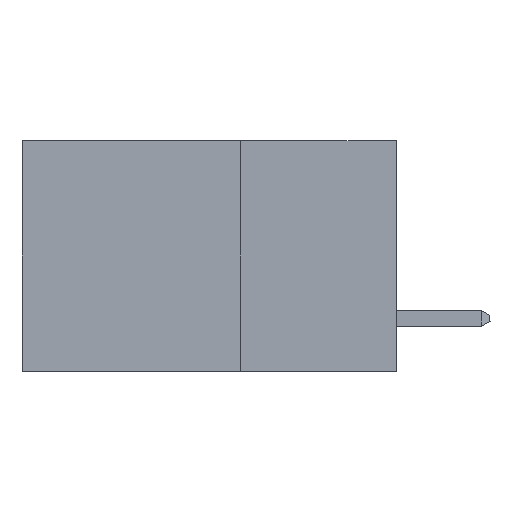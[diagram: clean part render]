
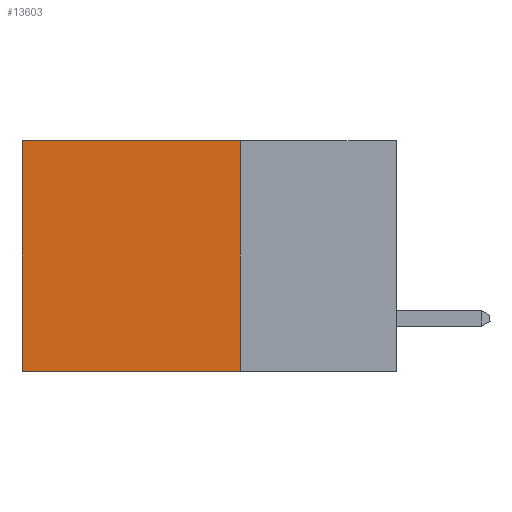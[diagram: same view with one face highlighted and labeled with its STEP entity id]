
A CAD part, left-side view. The second image highlights one B-rep face of the part: STEP entity #13603.
In plain terms, the highlighted planar face has unit normal (-1, 0, 0).
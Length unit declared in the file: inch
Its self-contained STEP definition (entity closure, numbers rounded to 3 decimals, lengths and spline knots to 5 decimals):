
#178 = VECTOR ( 'NONE', #5816, 39.37008 ) ;
#515 = EDGE_CURVE ( 'NONE', #1883, #13728, #14720, .T. ) ;
#1825 = VECTOR ( 'NONE', #14059, 39.37008 ) ;
#1883 = VERTEX_POINT ( 'NONE', #7323 ) ;
#2165 = CARTESIAN_POINT ( 'NONE',  ( 0.298, 0.6, -0.37 ) ) ;
#3033 = LINE ( 'NONE', #6489, #6186 ) ;
#3456 = EDGE_LOOP ( 'NONE', ( #7379, #7427, #7745, #8244 ) ) ;
#3916 = CARTESIAN_POINT ( 'NONE',  ( 0.298, 0.6, 0. ) ) ;
#4239 = CARTESIAN_POINT ( 'NONE',  ( 0.298, 0.6, 0. ) ) ;
#4866 = VECTOR ( 'NONE', #12327, 39.37008 ) ;
#5484 = EDGE_CURVE ( 'NONE', #1883, #8953, #9829, .T. ) ;
#5716 = VERTEX_POINT ( 'NONE', #2165 ) ;
#5816 = DIRECTION ( 'NONE',  ( 0., 0., -1. ) ) ;
#5829 = CARTESIAN_POINT ( 'NONE',  ( 0.298, 0.25, 0. ) ) ;
#6186 = VECTOR ( 'NONE', #14607, 39.37008 ) ;
#6489 = CARTESIAN_POINT ( 'NONE',  ( 0.298, 0.25, -0.37 ) ) ;
#6568 = EDGE_CURVE ( 'NONE', #13728, #5716, #11231, .T. ) ;
#7288 = DIRECTION ( 'NONE',  ( 0., 0., -1. ) ) ;
#7323 = CARTESIAN_POINT ( 'NONE',  ( 0.298, 0.25, 0. ) ) ;
#7379 = ORIENTED_EDGE ( 'NONE', *, *, #6568, .T. ) ;
#7427 = ORIENTED_EDGE ( 'NONE', *, *, #13308, .F. ) ;
#7745 = ORIENTED_EDGE ( 'NONE', *, *, #5484, .F. ) ;
#8244 = ORIENTED_EDGE ( 'NONE', *, *, #515, .T. ) ;
#8310 = AXIS2_PLACEMENT_3D ( 'NONE', #13139, #14270, #7288 ) ;
#8953 = VERTEX_POINT ( 'NONE', #9552 ) ;
#9552 = CARTESIAN_POINT ( 'NONE',  ( 0.298, 0.25, -0.37 ) ) ;
#9829 = LINE ( 'NONE', #5829, #178 ) ;
#11211 = FACE_OUTER_BOUND ( 'NONE', #3456, .T. ) ;
#11231 = LINE ( 'NONE', #4239, #4866 ) ;
#11995 = PLANE ( 'NONE',  #8310 ) ;
#12327 = DIRECTION ( 'NONE',  ( 0., 0., -1. ) ) ;
#13139 = CARTESIAN_POINT ( 'NONE',  ( 0.298, 0.25, 0. ) ) ;
#13308 = EDGE_CURVE ( 'NONE', #8953, #5716, #3033, .T. ) ;
#13603 = ADVANCED_FACE ( 'NONE', ( #11211 ), #11995, .F. ) ;
#13728 = VERTEX_POINT ( 'NONE', #3916 ) ;
#13765 = CARTESIAN_POINT ( 'NONE',  ( 0.298, 0.25, 0. ) ) ;
#14059 = DIRECTION ( 'NONE',  ( 0., 1., 0. ) ) ;
#14270 = DIRECTION ( 'NONE',  ( 1., 0., 0. ) ) ;
#14607 = DIRECTION ( 'NONE',  ( 0., 1., 0. ) ) ;
#14720 = LINE ( 'NONE', #13765, #1825 ) ;
